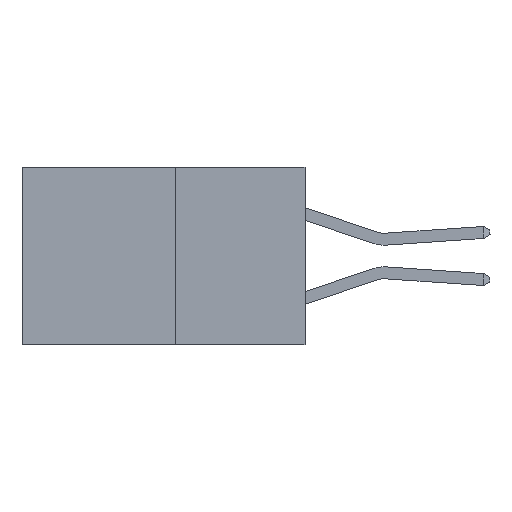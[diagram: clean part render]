
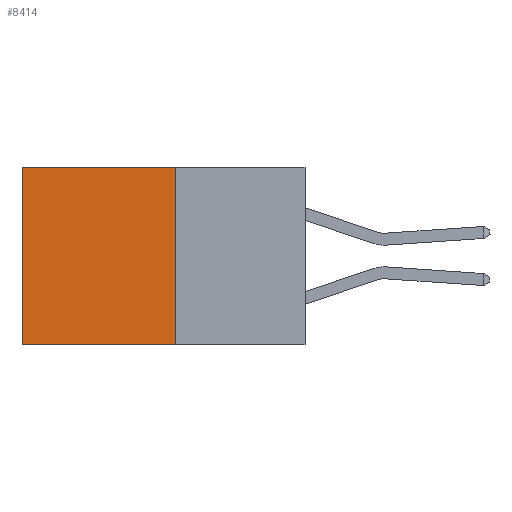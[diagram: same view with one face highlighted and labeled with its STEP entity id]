
A CAD part, left-side view. The second image highlights one B-rep face of the part: STEP entity #8414.
In plain terms, the highlighted planar face has unit normal (-1, 0, 0).
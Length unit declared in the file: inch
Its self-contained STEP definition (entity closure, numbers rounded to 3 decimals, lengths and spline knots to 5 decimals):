
#756 = EDGE_CURVE ( 'NONE', #11586, #4332, #19003, .T. ) ;
#1140 = DIRECTION ( 'NONE',  ( 1., 0., 0. ) ) ;
#1723 = DIRECTION ( 'NONE',  ( 0., 1., 0. ) ) ;
#2874 = ORIENTED_EDGE ( 'NONE', *, *, #756, .F. ) ;
#2890 = VERTEX_POINT ( 'NONE', #8883 ) ;
#3994 = DIRECTION ( 'NONE',  ( 0., 0., -1. ) ) ;
#4208 = CARTESIAN_POINT ( 'NONE',  ( 0.277, 0.59, -0.37 ) ) ;
#4269 = ORIENTED_EDGE ( 'NONE', *, *, #13800, .T. ) ;
#4332 = VERTEX_POINT ( 'NONE', #9523 ) ;
#4776 = DIRECTION ( 'NONE',  ( 0., 0., -1. ) ) ;
#6109 = CARTESIAN_POINT ( 'NONE',  ( 0.277, 0.27, -0.37 ) ) ;
#7159 = EDGE_LOOP ( 'NONE', ( #20958, #16314, #2874, #4269 ) ) ;
#7456 = LINE ( 'NONE', #15934, #20856 ) ;
#7537 = CARTESIAN_POINT ( 'NONE',  ( 0.277, 0.27, -0.37 ) ) ;
#8414 = ADVANCED_FACE ( 'NONE', ( #11129 ), #10879, .F. ) ;
#8589 = EDGE_CURVE ( 'NONE', #4332, #2890, #20938, .T. ) ;
#8883 = CARTESIAN_POINT ( 'NONE',  ( 0.277, 0.59, -0.37 ) ) ;
#9523 = CARTESIAN_POINT ( 'NONE',  ( 0.277, 0.27, -0.37 ) ) ;
#9907 = DIRECTION ( 'NONE',  ( 0., 1., 0. ) ) ;
#9925 = VECTOR ( 'NONE', #3994, 39.37008 ) ;
#10080 = VECTOR ( 'NONE', #4776, 39.37008 ) ;
#10396 = DIRECTION ( 'NONE',  ( 0., 0., -1. ) ) ;
#10879 = PLANE ( 'NONE',  #11050 ) ;
#11020 = CARTESIAN_POINT ( 'NONE',  ( 0.277, 0.59, 0. ) ) ;
#11050 = AXIS2_PLACEMENT_3D ( 'NONE', #13766, #1140, #10396 ) ;
#11129 = FACE_OUTER_BOUND ( 'NONE', #7159, .T. ) ;
#11586 = VERTEX_POINT ( 'NONE', #18512 ) ;
#12390 = VECTOR ( 'NONE', #1723, 39.37008 ) ;
#13766 = CARTESIAN_POINT ( 'NONE',  ( 0.277, 0.27, -0.37 ) ) ;
#13800 = EDGE_CURVE ( 'NONE', #11586, #17486, #7456, .T. ) ;
#15934 = CARTESIAN_POINT ( 'NONE',  ( 0.277, 0.27, 0. ) ) ;
#16314 = ORIENTED_EDGE ( 'NONE', *, *, #8589, .F. ) ;
#17486 = VERTEX_POINT ( 'NONE', #11020 ) ;
#18512 = CARTESIAN_POINT ( 'NONE',  ( 0.277, 0.27, 0. ) ) ;
#18621 = EDGE_CURVE ( 'NONE', #17486, #2890, #19162, .T. ) ;
#19003 = LINE ( 'NONE', #6109, #9925 ) ;
#19162 = LINE ( 'NONE', #4208, #10080 ) ;
#20856 = VECTOR ( 'NONE', #9907, 39.37008 ) ;
#20938 = LINE ( 'NONE', #7537, #12390 ) ;
#20958 = ORIENTED_EDGE ( 'NONE', *, *, #18621, .T. ) ;
